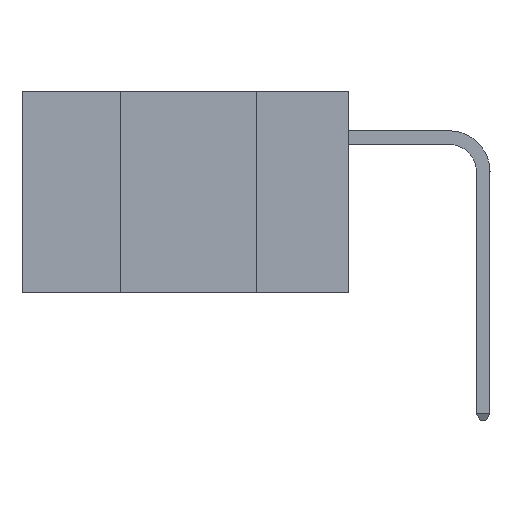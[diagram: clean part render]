
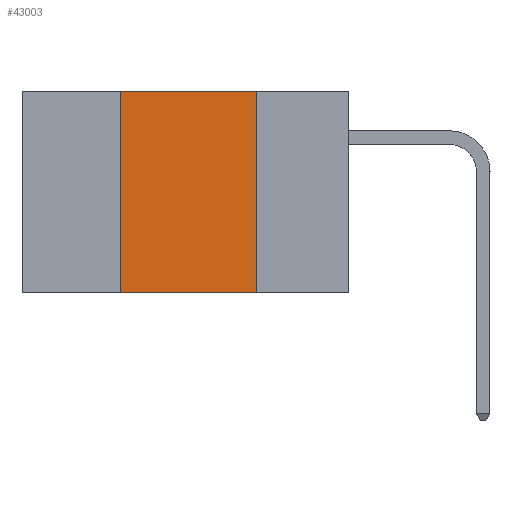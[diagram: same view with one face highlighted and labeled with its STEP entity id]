
A CAD part, left-side view. The second image highlights one B-rep face of the part: STEP entity #43003.
In plain terms, the highlighted planar face has unit normal (-1, 0, 0).
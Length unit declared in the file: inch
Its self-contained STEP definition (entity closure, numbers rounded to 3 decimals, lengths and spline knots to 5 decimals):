
#770 = CARTESIAN_POINT ( 'NONE',  ( 0., 0.17, -0.37 ) ) ;
#1870 = EDGE_CURVE ( 'NONE', #36663, #5343, #30175, .T. ) ;
#1872 = ORIENTED_EDGE ( 'NONE', *, *, #43960, .F. ) ;
#1878 = LINE ( 'NONE', #30362, #38966 ) ;
#2994 = DIRECTION ( 'NONE',  ( 0., -1., 0. ) ) ;
#3585 = EDGE_CURVE ( 'NONE', #44744, #35167, #1878, .T. ) ;
#5343 = VERTEX_POINT ( 'NONE', #770 ) ;
#6315 = CARTESIAN_POINT ( 'NONE',  ( 0., 0.6, -0.37 ) ) ;
#6704 = AXIS2_PLACEMENT_3D ( 'NONE', #32034, #17756, #24656 ) ;
#6899 = LINE ( 'NONE', #43026, #31644 ) ;
#7692 = VECTOR ( 'NONE', #2994, 39.37008 ) ;
#8734 = CARTESIAN_POINT ( 'NONE',  ( 0., 0.17, 0. ) ) ;
#12265 = ORIENTED_EDGE ( 'NONE', *, *, #15988, .F. ) ;
#15988 = EDGE_CURVE ( 'NONE', #36663, #44744, #6899, .T. ) ;
#17756 = DIRECTION ( 'NONE',  ( 1., 0., 0. ) ) ;
#21398 = CARTESIAN_POINT ( 'NONE',  ( 0., 0.42, 0. ) ) ;
#23285 = DIRECTION ( 'NONE',  ( 0., -1., 0. ) ) ;
#24520 = DIRECTION ( 'NONE',  ( 0., 0., 1. ) ) ;
#24656 = DIRECTION ( 'NONE',  ( 0., 0., -1. ) ) ;
#24702 = VECTOR ( 'NONE', #31233, 39.37008 ) ;
#28754 = PLANE ( 'NONE',  #6704 ) ;
#30175 = LINE ( 'NONE', #6315, #7692 ) ;
#30362 = CARTESIAN_POINT ( 'NONE',  ( 0., 0.6, 0. ) ) ;
#30582 = ORIENTED_EDGE ( 'NONE', *, *, #3585, .F. ) ;
#31233 = DIRECTION ( 'NONE',  ( 0., 0., -1. ) ) ;
#31644 = VECTOR ( 'NONE', #24520, 39.37008 ) ;
#32034 = CARTESIAN_POINT ( 'NONE',  ( 0., 0.6, 0. ) ) ;
#34800 = LINE ( 'NONE', #41577, #24702 ) ;
#35167 = VERTEX_POINT ( 'NONE', #8734 ) ;
#35633 = EDGE_LOOP ( 'NONE', ( #1872, #30582, #12265, #46484 ) ) ;
#36663 = VERTEX_POINT ( 'NONE', #38508 ) ;
#38508 = CARTESIAN_POINT ( 'NONE',  ( 0., 0.42, -0.37 ) ) ;
#38966 = VECTOR ( 'NONE', #23285, 39.37008 ) ;
#41248 = FACE_OUTER_BOUND ( 'NONE', #35633, .T. ) ;
#41577 = CARTESIAN_POINT ( 'NONE',  ( 0., 0.17, 0. ) ) ;
#43003 = ADVANCED_FACE ( 'NONE', ( #41248 ), #28754, .F. ) ;
#43026 = CARTESIAN_POINT ( 'NONE',  ( 0., 0.42, 0. ) ) ;
#43960 = EDGE_CURVE ( 'NONE', #35167, #5343, #34800, .T. ) ;
#44744 = VERTEX_POINT ( 'NONE', #21398 ) ;
#46484 = ORIENTED_EDGE ( 'NONE', *, *, #1870, .T. ) ;
